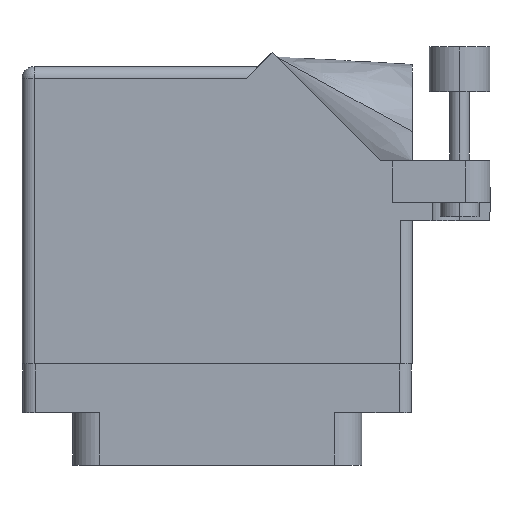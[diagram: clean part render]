
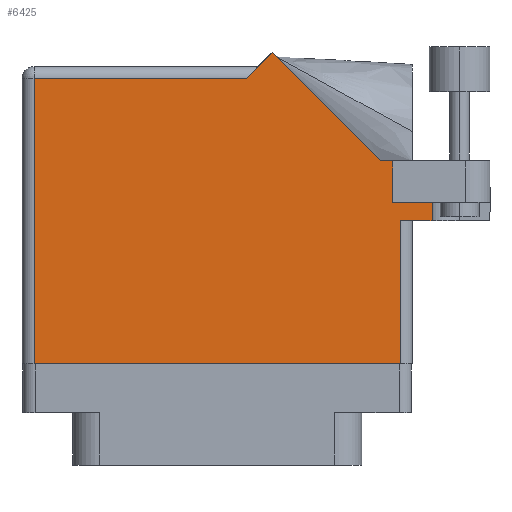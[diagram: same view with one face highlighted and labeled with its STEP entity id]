
A CAD part, front view. The second image highlights one B-rep face of the part: STEP entity #6425.
In plain terms, the highlighted face is planar.
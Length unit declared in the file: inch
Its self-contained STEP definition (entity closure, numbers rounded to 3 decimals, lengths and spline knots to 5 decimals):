
#7 = CARTESIAN_POINT ( 'NONE',  ( -1.005, 1.368, 0.455 ) ) ;
#1005 = VERTEX_POINT ( 'NONE', #10322 ) ;
#1144 = ORIENTED_EDGE ( 'NONE', *, *, #38041, .T. ) ;
#1575 = CARTESIAN_POINT ( 'NONE',  ( -0.943, -0.1, 0.455 ) ) ;
#1936 = DIRECTION ( 'NONE',  ( -0.707, 0.707, 0. ) ) ;
#2207 = CARTESIAN_POINT ( 'NONE',  ( 1.1065, 0.731, 0.455 ) ) ;
#2270 = EDGE_CURVE ( 'NONE', #33466, #5023, #2858, .T. ) ;
#2444 = DIRECTION ( 'NONE',  ( -1., 0., 0. ) ) ;
#2858 = LINE ( 'NONE', #1575, #20011 ) ;
#3530 = VECTOR ( 'NONE', #1936, 39.37008 ) ;
#3572 = EDGE_CURVE ( 'NONE', #13174, #12551, #10062, .T. ) ;
#3960 = CARTESIAN_POINT ( 'NONE',  ( 0.905, 0.731, 0.455 ) ) ;
#4724 = CARTESIAN_POINT ( 'NONE',  ( 0.212, 1.43, 0.455 ) ) ;
#5023 = VERTEX_POINT ( 'NONE', #29189 ) ;
#5603 = EDGE_CURVE ( 'NONE', #12551, #27628, #27230, .T. ) ;
#6425 = ADVANCED_FACE ( 'NONE', ( #29206 ), #27226, .F. ) ;
#6723 = EDGE_CURVE ( 'NONE', #13174, #17992, #34539, .T. ) ;
#7029 = EDGE_CURVE ( 'NONE', #5023, #29043, #19803, .T. ) ;
#8365 = CARTESIAN_POINT ( 'NONE',  ( 1.1065, 1.06177, 0.455 ) ) ;
#8790 = VECTOR ( 'NONE', #29919, 39.37008 ) ;
#9943 = DIRECTION ( 'NONE',  ( 1., 0., 0. ) ) ;
#10062 = LINE ( 'NONE', #15037, #28221 ) ;
#10084 = ORIENTED_EDGE ( 'NONE', *, *, #6723, .F. ) ;
#10258 = LINE ( 'NONE', #39613, #8790 ) ;
#10322 = CARTESIAN_POINT ( 'NONE',  ( 1.1065, 0.637, 0.455 ) ) ;
#11231 = DIRECTION ( 'NONE',  ( 0., -1., 0. ) ) ;
#11467 = VECTOR ( 'NONE', #21466, 39.37008 ) ;
#11554 = EDGE_CURVE ( 'NONE', #28956, #33466, #26906, .T. ) ;
#11759 = DIRECTION ( 'NONE',  ( 0., 1., 0. ) ) ;
#11832 = VECTOR ( 'NONE', #11231, 39.37008 ) ;
#12551 = VERTEX_POINT ( 'NONE', #17561 ) ;
#13174 = VERTEX_POINT ( 'NONE', #40509 ) ;
#13525 = CARTESIAN_POINT ( 'NONE',  ( 0.15, 1.368, 0.455 ) ) ;
#15037 = CARTESIAN_POINT ( 'NONE',  ( 0.905, 0.731, 0.455 ) ) ;
#15126 = CARTESIAN_POINT ( 'NONE',  ( -1.005, -0.1, 0.455 ) ) ;
#15289 = EDGE_CURVE ( 'NONE', #17992, #1005, #35820, .T. ) ;
#15354 = EDGE_CURVE ( 'NONE', #27628, #23660, #16719, .T. ) ;
#16719 = LINE ( 'NONE', #20702, #3530 ) ;
#16896 = VECTOR ( 'NONE', #9943, 39.37008 ) ;
#17361 = DIRECTION ( 'NONE',  ( -1., 0., 0. ) ) ;
#17561 = CARTESIAN_POINT ( 'NONE',  ( 0.905, 0.944, 0.455 ) ) ;
#17992 = VERTEX_POINT ( 'NONE', #2207 ) ;
#19803 = LINE ( 'NONE', #15126, #11467 ) ;
#20011 = VECTOR ( 'NONE', #36061, 39.37008 ) ;
#20702 = CARTESIAN_POINT ( 'NONE',  ( 0.83942, 0.944, 0.455 ) ) ;
#21281 = ORIENTED_EDGE ( 'NONE', *, *, #5603, .T. ) ;
#21466 = DIRECTION ( 'NONE',  ( 1., 0., 0. ) ) ;
#21621 = EDGE_CURVE ( 'NONE', #40206, #1005, #27388, .T. ) ;
#21993 = EDGE_LOOP ( 'NONE', ( #34818, #1144, #37782, #24222, #10084, #33987, #21281, #27966, #34368, #30321, #22087 ) ) ;
#22087 = ORIENTED_EDGE ( 'NONE', *, *, #2270, .T. ) ;
#22163 = CARTESIAN_POINT ( 'NONE',  ( -0.943, 1.368, 0.455 ) ) ;
#22189 = DIRECTION ( 'NONE',  ( -1., 0., 0. ) ) ;
#23660 = VERTEX_POINT ( 'NONE', #26738 ) ;
#24222 = ORIENTED_EDGE ( 'NONE', *, *, #15289, .F. ) ;
#26637 = CARTESIAN_POINT ( 'NONE',  ( 1.005, 0.637, 0.455 ) ) ;
#26738 = CARTESIAN_POINT ( 'NONE',  ( 0.28271, 1.50071, 0.455 ) ) ;
#26906 = LINE ( 'NONE', #7, #31336 ) ;
#27226 = PLANE ( 'NONE',  #28970 ) ;
#27230 = LINE ( 'NONE', #29989, #30244 ) ;
#27388 = LINE ( 'NONE', #26637, #39157 ) ;
#27628 = VERTEX_POINT ( 'NONE', #31931 ) ;
#27966 = ORIENTED_EDGE ( 'NONE', *, *, #15354, .T. ) ;
#28221 = VECTOR ( 'NONE', #11759, 39.37008 ) ;
#28956 = VERTEX_POINT ( 'NONE', #13525 ) ;
#28970 = AXIS2_PLACEMENT_3D ( 'NONE', #35988, #36524, #17361 ) ;
#29043 = VERTEX_POINT ( 'NONE', #39270 ) ;
#29189 = CARTESIAN_POINT ( 'NONE',  ( -0.943, -0.1, 0.455 ) ) ;
#29206 = FACE_OUTER_BOUND ( 'NONE', #21993, .T. ) ;
#29662 = EDGE_CURVE ( 'NONE', #23660, #28956, #39236, .T. ) ;
#29919 = DIRECTION ( 'NONE',  ( 0., 1., 0. ) ) ;
#29989 = CARTESIAN_POINT ( 'NONE',  ( 1.405, 0.944, 0.455 ) ) ;
#30244 = VECTOR ( 'NONE', #2444, 39.37008 ) ;
#30321 = ORIENTED_EDGE ( 'NONE', *, *, #11554, .T. ) ;
#31336 = VECTOR ( 'NONE', #22189, 39.37008 ) ;
#31345 = VECTOR ( 'NONE', #33183, 39.37008 ) ;
#31931 = CARTESIAN_POINT ( 'NONE',  ( 0.83942, 0.944, 0.455 ) ) ;
#33183 = DIRECTION ( 'NONE',  ( -0.707, -0.707, 0. ) ) ;
#33466 = VERTEX_POINT ( 'NONE', #22163 ) ;
#33987 = ORIENTED_EDGE ( 'NONE', *, *, #3572, .T. ) ;
#34368 = ORIENTED_EDGE ( 'NONE', *, *, #29662, .T. ) ;
#34539 = LINE ( 'NONE', #3960, #16896 ) ;
#34818 = ORIENTED_EDGE ( 'NONE', *, *, #7029, .T. ) ;
#35820 = LINE ( 'NONE', #8365, #11832 ) ;
#35988 = CARTESIAN_POINT ( 'NONE',  ( -1.005, 1.43, 0.455 ) ) ;
#36061 = DIRECTION ( 'NONE',  ( 0., -1., 0. ) ) ;
#36080 = DIRECTION ( 'NONE',  ( 1., 0., 0. ) ) ;
#36524 = DIRECTION ( 'NONE',  ( 0., 0., -1. ) ) ;
#37484 = CARTESIAN_POINT ( 'NONE',  ( 0.943, 0.637, 0.455 ) ) ;
#37782 = ORIENTED_EDGE ( 'NONE', *, *, #21621, .T. ) ;
#38041 = EDGE_CURVE ( 'NONE', #29043, #40206, #10258, .T. ) ;
#39157 = VECTOR ( 'NONE', #36080, 39.37008 ) ;
#39236 = LINE ( 'NONE', #4724, #31345 ) ;
#39270 = CARTESIAN_POINT ( 'NONE',  ( 0.943, -0.1, 0.455 ) ) ;
#39613 = CARTESIAN_POINT ( 'NONE',  ( 0.943, 0.637, 0.455 ) ) ;
#40206 = VERTEX_POINT ( 'NONE', #37484 ) ;
#40509 = CARTESIAN_POINT ( 'NONE',  ( 0.905, 0.731, 0.455 ) ) ;
